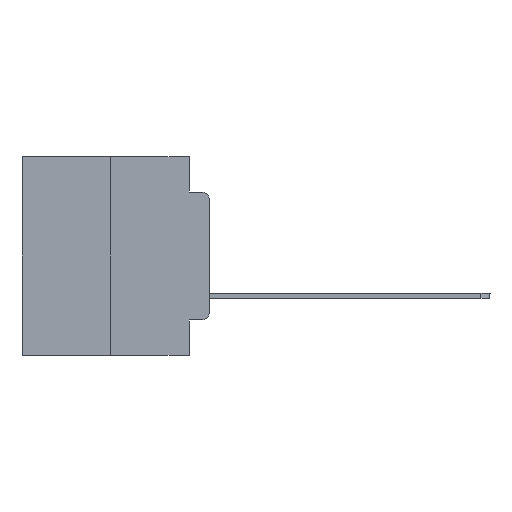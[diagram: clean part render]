
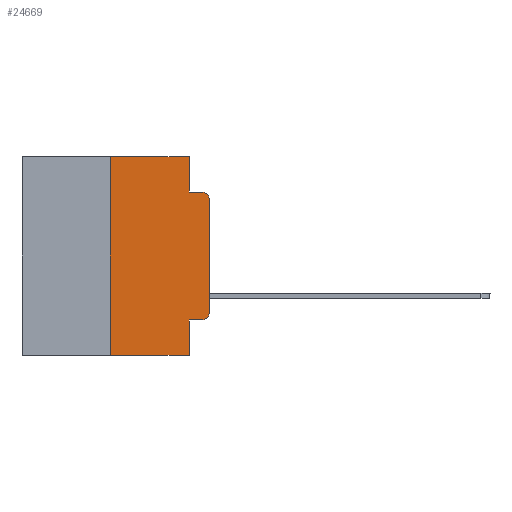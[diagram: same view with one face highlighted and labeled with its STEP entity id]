
A CAD part, left-side view. The second image highlights one B-rep face of the part: STEP entity #24669.
In plain terms, the highlighted planar face has unit normal (-1, 0, 0).
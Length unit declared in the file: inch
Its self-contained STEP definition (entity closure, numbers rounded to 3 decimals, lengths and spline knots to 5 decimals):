
#626 = CARTESIAN_POINT ( 'NONE',  ( 0., 0.25, 0. ) ) ;
#792 = VERTEX_POINT ( 'NONE', #21572 ) ;
#1256 = AXIS2_PLACEMENT_3D ( 'NONE', #2444, #16714, #4507 ) ;
#1262 = LINE ( 'NONE', #8790, #15941 ) ;
#2146 = EDGE_LOOP ( 'NONE', ( #10842, #11618, #4519, #22401, #25276, #10530, #14309, #21464, #14334, #21731 ) ) ;
#2444 = CARTESIAN_POINT ( 'NONE',  ( 0., 0.02, -0.1085 ) ) ;
#2900 = EDGE_CURVE ( 'NONE', #17110, #23707, #22388, .T. ) ;
#3763 = VERTEX_POINT ( 'NONE', #626 ) ;
#3804 = VERTEX_POINT ( 'NONE', #22929 ) ;
#3953 = VERTEX_POINT ( 'NONE', #11395 ) ;
#4481 = VERTEX_POINT ( 'NONE', #23062 ) ;
#4507 = DIRECTION ( 'NONE',  ( 0., 0., -1. ) ) ;
#4519 = ORIENTED_EDGE ( 'NONE', *, *, #25768, .F. ) ;
#4596 = CARTESIAN_POINT ( 'NONE',  ( 0., 0., 0. ) ) ;
#5587 = CARTESIAN_POINT ( 'NONE',  ( 0., 0.051, 0. ) ) ;
#5978 = EDGE_CURVE ( 'NONE', #15955, #3763, #16455, .T. ) ;
#6045 = VECTOR ( 'NONE', #12303, 39.37008 ) ;
#6098 = VECTOR ( 'NONE', #7485, 39.37008 ) ;
#6292 = CARTESIAN_POINT ( 'NONE',  ( 0., 0.051, -0.0885 ) ) ;
#6401 = EDGE_CURVE ( 'NONE', #3953, #3804, #18967, .T. ) ;
#7229 = CARTESIAN_POINT ( 'NONE',  ( 0., 0.051, -0.4115 ) ) ;
#7485 = DIRECTION ( 'NONE',  ( 0., -1., 0. ) ) ;
#7616 = DIRECTION ( 'NONE',  ( 0., 0., -1. ) ) ;
#8623 = DIRECTION ( 'NONE',  ( 0., -1., 0. ) ) ;
#8790 = CARTESIAN_POINT ( 'NONE',  ( 0., 0.473, 0. ) ) ;
#9276 = DIRECTION ( 'NONE',  ( -1., 0., 0. ) ) ;
#9376 = CARTESIAN_POINT ( 'NONE',  ( 0., 0.473, -0.5 ) ) ;
#9392 = CARTESIAN_POINT ( 'NONE',  ( 0., 0.02, -0.4115 ) ) ;
#9808 = CARTESIAN_POINT ( 'NONE',  ( 0., 0.051, 0. ) ) ;
#10507 = VECTOR ( 'NONE', #24884, 39.37008 ) ;
#10530 = ORIENTED_EDGE ( 'NONE', *, *, #5978, .F. ) ;
#10842 = ORIENTED_EDGE ( 'NONE', *, *, #14105, .T. ) ;
#11395 = CARTESIAN_POINT ( 'NONE',  ( 0., 0.051, 0. ) ) ;
#11538 = CARTESIAN_POINT ( 'NONE',  ( 0., 0., -0.3915 ) ) ;
#11564 = CARTESIAN_POINT ( 'NONE',  ( 0., 0.051, -0.4115 ) ) ;
#11618 = ORIENTED_EDGE ( 'NONE', *, *, #16920, .T. ) ;
#12022 = CIRCLE ( 'NONE', #1256, 0.02 ) ;
#12185 = LINE ( 'NONE', #9376, #6098 ) ;
#12303 = DIRECTION ( 'NONE',  ( 0., -1., 0. ) ) ;
#12522 = LINE ( 'NONE', #7229, #22656 ) ;
#12994 = LINE ( 'NONE', #9808, #14310 ) ;
#13269 = VECTOR ( 'NONE', #7616, 39.37008 ) ;
#14105 = EDGE_CURVE ( 'NONE', #23707, #4481, #24800, .T. ) ;
#14309 = ORIENTED_EDGE ( 'NONE', *, *, #24873, .T. ) ;
#14310 = VECTOR ( 'NONE', #20059, 39.37008 ) ;
#14334 = ORIENTED_EDGE ( 'NONE', *, *, #24843, .T. ) ;
#15614 = CARTESIAN_POINT ( 'NONE',  ( 0., 0.02, -0.3915 ) ) ;
#15667 = FACE_OUTER_BOUND ( 'NONE', #2146, .T. ) ;
#15825 = VECTOR ( 'NONE', #18380, 39.37008 ) ;
#15941 = VECTOR ( 'NONE', #8623, 39.37008 ) ;
#15955 = VERTEX_POINT ( 'NONE', #23503 ) ;
#16455 = LINE ( 'NONE', #20174, #15825 ) ;
#16714 = DIRECTION ( 'NONE',  ( -1., 0., 0. ) ) ;
#16920 = EDGE_CURVE ( 'NONE', #4481, #21323, #12022, .T. ) ;
#16938 = PLANE ( 'NONE',  #21715 ) ;
#17110 = VERTEX_POINT ( 'NONE', #9392 ) ;
#18161 = LINE ( 'NONE', #6292, #6045 ) ;
#18380 = DIRECTION ( 'NONE',  ( 0., 0., 1. ) ) ;
#18967 = LINE ( 'NONE', #5587, #13269 ) ;
#18990 = DIRECTION ( 'NONE',  ( 1., 0., 0. ) ) ;
#19081 = DIRECTION ( 'NONE',  ( 0., 0., -1. ) ) ;
#19525 = DIRECTION ( 'NONE',  ( 0., -1., 0. ) ) ;
#20059 = DIRECTION ( 'NONE',  ( 0., 0., -1. ) ) ;
#20174 = CARTESIAN_POINT ( 'NONE',  ( 0., 0.25, 0. ) ) ;
#20815 = AXIS2_PLACEMENT_3D ( 'NONE', #15614, #9276, #25560 ) ;
#21323 = VERTEX_POINT ( 'NONE', #25458 ) ;
#21464 = ORIENTED_EDGE ( 'NONE', *, *, #22096, .F. ) ;
#21572 = CARTESIAN_POINT ( 'NONE',  ( 0., 0.051, -0.5 ) ) ;
#21715 = AXIS2_PLACEMENT_3D ( 'NONE', #25375, #18990, #19081 ) ;
#21731 = ORIENTED_EDGE ( 'NONE', *, *, #2900, .T. ) ;
#22096 = EDGE_CURVE ( 'NONE', #26217, #792, #12994, .T. ) ;
#22388 = CIRCLE ( 'NONE', #20815, 0.02 ) ;
#22401 = ORIENTED_EDGE ( 'NONE', *, *, #6401, .F. ) ;
#22656 = VECTOR ( 'NONE', #19525, 39.37008 ) ;
#22929 = CARTESIAN_POINT ( 'NONE',  ( 0., 0.051, -0.0885 ) ) ;
#23062 = CARTESIAN_POINT ( 'NONE',  ( 0., 0., -0.1085 ) ) ;
#23503 = CARTESIAN_POINT ( 'NONE',  ( 0., 0.25, -0.5 ) ) ;
#23707 = VERTEX_POINT ( 'NONE', #11538 ) ;
#24669 = ADVANCED_FACE ( 'NONE', ( #15667 ), #16938, .F. ) ;
#24800 = LINE ( 'NONE', #4596, #10507 ) ;
#24843 = EDGE_CURVE ( 'NONE', #26217, #17110, #12522, .T. ) ;
#24873 = EDGE_CURVE ( 'NONE', #15955, #792, #12185, .T. ) ;
#24884 = DIRECTION ( 'NONE',  ( 0., 0., 1. ) ) ;
#25276 = ORIENTED_EDGE ( 'NONE', *, *, #25298, .F. ) ;
#25298 = EDGE_CURVE ( 'NONE', #3763, #3953, #1262, .T. ) ;
#25375 = CARTESIAN_POINT ( 'NONE',  ( 0., 0.473, 0. ) ) ;
#25458 = CARTESIAN_POINT ( 'NONE',  ( 0., 0.02, -0.0885 ) ) ;
#25560 = DIRECTION ( 'NONE',  ( 0., 0., -1. ) ) ;
#25768 = EDGE_CURVE ( 'NONE', #3804, #21323, #18161, .T. ) ;
#26217 = VERTEX_POINT ( 'NONE', #11564 ) ;
